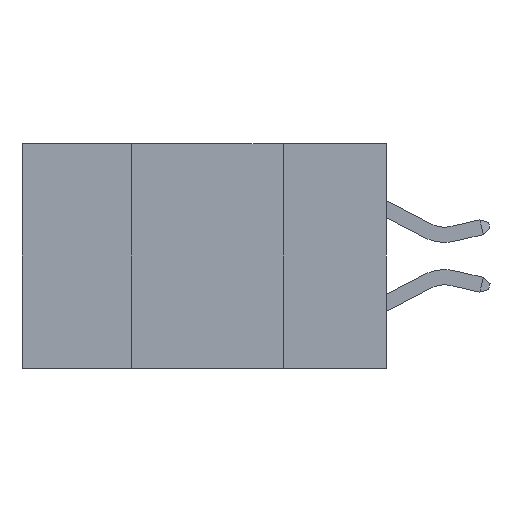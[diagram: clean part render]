
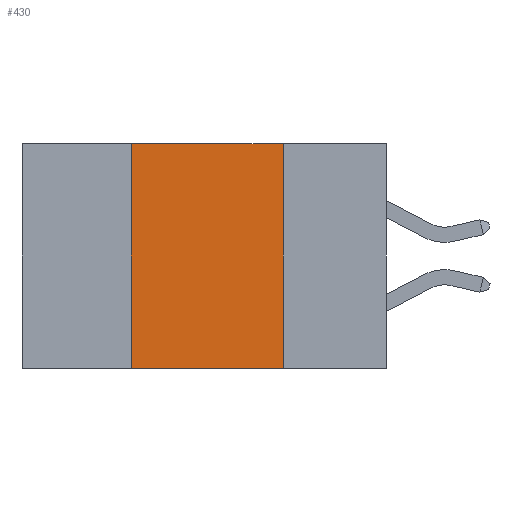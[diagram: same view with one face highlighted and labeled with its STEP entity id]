
A CAD part, left-side view. The second image highlights one B-rep face of the part: STEP entity #430.
In plain terms, the highlighted planar face has unit normal (-1, 0, 0).
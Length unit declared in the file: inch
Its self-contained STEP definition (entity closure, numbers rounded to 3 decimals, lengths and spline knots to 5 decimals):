
#194 = VECTOR ( 'NONE', #6108, 39.37008 ) ;
#430 = ADVANCED_FACE ( 'NONE', ( #16751 ), #4115, .F. ) ;
#865 = VECTOR ( 'NONE', #2325, 39.37008 ) ;
#1610 = EDGE_CURVE ( 'NONE', #16192, #15186, #8489, .T. ) ;
#2141 = VERTEX_POINT ( 'NONE', #16350 ) ;
#2152 = EDGE_CURVE ( 'NONE', #2141, #4069, #5889, .T. ) ;
#2325 = DIRECTION ( 'NONE',  ( 0., -1., 0. ) ) ;
#2559 = CARTESIAN_POINT ( 'NONE',  ( 0., 0.17, 0. ) ) ;
#2841 = EDGE_CURVE ( 'NONE', #4069, #15186, #15400, .T. ) ;
#3032 = CARTESIAN_POINT ( 'NONE',  ( 0., 0.17, 0. ) ) ;
#3879 = CARTESIAN_POINT ( 'NONE',  ( 0., 0.6, 0. ) ) ;
#3950 = CARTESIAN_POINT ( 'NONE',  ( 0., 0.42, -0.37 ) ) ;
#4069 = VERTEX_POINT ( 'NONE', #2559 ) ;
#4115 = PLANE ( 'NONE',  #10798 ) ;
#4424 = ORIENTED_EDGE ( 'NONE', *, *, #2841, .F. ) ;
#5889 = LINE ( 'NONE', #3879, #8491 ) ;
#6108 = DIRECTION ( 'NONE',  ( 0., 0., 1. ) ) ;
#6178 = ORIENTED_EDGE ( 'NONE', *, *, #1610, .T. ) ;
#6612 = DIRECTION ( 'NONE',  ( 0., -1., 0. ) ) ;
#8287 = DIRECTION ( 'NONE',  ( 0., 0., -1. ) ) ;
#8458 = LINE ( 'NONE', #17310, #194 ) ;
#8489 = LINE ( 'NONE', #9471, #865 ) ;
#8491 = VECTOR ( 'NONE', #6612, 39.37008 ) ;
#9471 = CARTESIAN_POINT ( 'NONE',  ( 0., 0.6, -0.37 ) ) ;
#9514 = DIRECTION ( 'NONE',  ( 1., 0., 0. ) ) ;
#9962 = DIRECTION ( 'NONE',  ( 0., 0., -1. ) ) ;
#10798 = AXIS2_PLACEMENT_3D ( 'NONE', #16475, #9514, #8287 ) ;
#11739 = CARTESIAN_POINT ( 'NONE',  ( 0., 0.17, -0.37 ) ) ;
#11740 = VECTOR ( 'NONE', #9962, 39.37008 ) ;
#12005 = EDGE_LOOP ( 'NONE', ( #4424, #13557, #15640, #6178 ) ) ;
#13557 = ORIENTED_EDGE ( 'NONE', *, *, #2152, .F. ) ;
#15186 = VERTEX_POINT ( 'NONE', #11739 ) ;
#15400 = LINE ( 'NONE', #3032, #11740 ) ;
#15640 = ORIENTED_EDGE ( 'NONE', *, *, #17284, .F. ) ;
#16192 = VERTEX_POINT ( 'NONE', #3950 ) ;
#16350 = CARTESIAN_POINT ( 'NONE',  ( 0., 0.42, 0. ) ) ;
#16475 = CARTESIAN_POINT ( 'NONE',  ( 0., 0.6, 0. ) ) ;
#16751 = FACE_OUTER_BOUND ( 'NONE', #12005, .T. ) ;
#17284 = EDGE_CURVE ( 'NONE', #16192, #2141, #8458, .T. ) ;
#17310 = CARTESIAN_POINT ( 'NONE',  ( 0., 0.42, 0. ) ) ;
